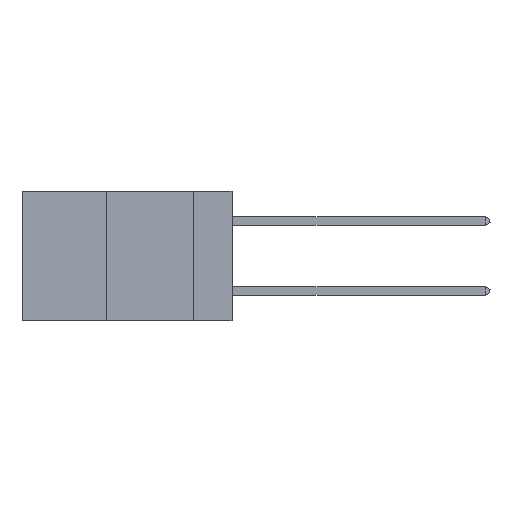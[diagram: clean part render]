
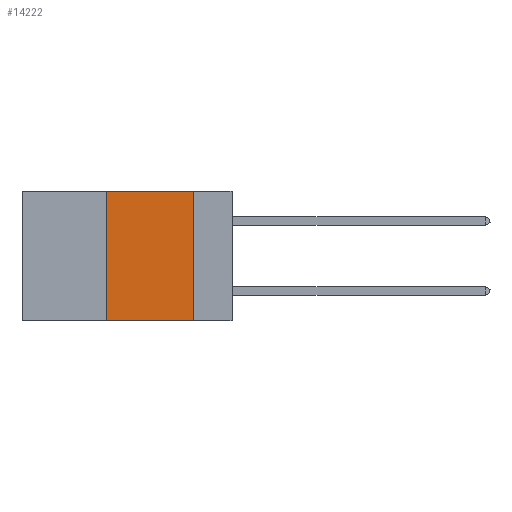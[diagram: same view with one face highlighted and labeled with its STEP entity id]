
A CAD part, left-side view. The second image highlights one B-rep face of the part: STEP entity #14222.
In plain terms, the highlighted planar face has unit normal (-1, 0, 0).
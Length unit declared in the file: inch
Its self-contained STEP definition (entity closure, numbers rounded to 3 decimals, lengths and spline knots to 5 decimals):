
#1043 = VECTOR ( 'NONE', #18296, 39.37008 ) ;
#1651 = CARTESIAN_POINT ( 'NONE',  ( 0., 0.11, 0. ) ) ;
#2403 = DIRECTION ( 'NONE',  ( 0., 0., 1. ) ) ;
#2477 = DIRECTION ( 'NONE',  ( 1., 0., 0. ) ) ;
#3644 = EDGE_CURVE ( 'NONE', #19221, #15955, #5813, .T. ) ;
#4206 = PLANE ( 'NONE',  #4920 ) ;
#4920 = AXIS2_PLACEMENT_3D ( 'NONE', #13035, #2477, #14788 ) ;
#5813 = LINE ( 'NONE', #13084, #1043 ) ;
#5834 = EDGE_CURVE ( 'NONE', #15955, #10063, #16811, .T. ) ;
#6502 = CARTESIAN_POINT ( 'NONE',  ( 0., 0.36, -0.37 ) ) ;
#8186 = DIRECTION ( 'NONE',  ( 0., -1., 0. ) ) ;
#8489 = VECTOR ( 'NONE', #2403, 39.37008 ) ;
#8500 = EDGE_CURVE ( 'NONE', #8532, #10063, #19958, .T. ) ;
#8532 = VERTEX_POINT ( 'NONE', #6502 ) ;
#8647 = VECTOR ( 'NONE', #9045, 39.37008 ) ;
#9045 = DIRECTION ( 'NONE',  ( 0., 0., -1. ) ) ;
#9354 = ORIENTED_EDGE ( 'NONE', *, *, #3644, .F. ) ;
#10063 = VERTEX_POINT ( 'NONE', #14155 ) ;
#11150 = ORIENTED_EDGE ( 'NONE', *, *, #5834, .F. ) ;
#11214 = CARTESIAN_POINT ( 'NONE',  ( 0., 0.36, 0. ) ) ;
#11793 = ORIENTED_EDGE ( 'NONE', *, *, #8500, .T. ) ;
#12041 = FACE_OUTER_BOUND ( 'NONE', #12995, .T. ) ;
#12995 = EDGE_LOOP ( 'NONE', ( #11150, #9354, #22563, #11793 ) ) ;
#13035 = CARTESIAN_POINT ( 'NONE',  ( 0., 0.6, 0. ) ) ;
#13084 = CARTESIAN_POINT ( 'NONE',  ( 0., 0.6, 0. ) ) ;
#14155 = CARTESIAN_POINT ( 'NONE',  ( 0., 0.11, -0.37 ) ) ;
#14199 = EDGE_CURVE ( 'NONE', #8532, #19221, #22297, .T. ) ;
#14222 = ADVANCED_FACE ( 'NONE', ( #12041 ), #4206, .F. ) ;
#14788 = DIRECTION ( 'NONE',  ( 0., 0., -1. ) ) ;
#15940 = VECTOR ( 'NONE', #8186, 39.37008 ) ;
#15955 = VERTEX_POINT ( 'NONE', #1651 ) ;
#16811 = LINE ( 'NONE', #21203, #8647 ) ;
#18296 = DIRECTION ( 'NONE',  ( 0., -1., 0. ) ) ;
#18586 = CARTESIAN_POINT ( 'NONE',  ( 0., 0.6, -0.37 ) ) ;
#19221 = VERTEX_POINT ( 'NONE', #20807 ) ;
#19958 = LINE ( 'NONE', #18586, #15940 ) ;
#20807 = CARTESIAN_POINT ( 'NONE',  ( 0., 0.36, 0. ) ) ;
#21203 = CARTESIAN_POINT ( 'NONE',  ( 0., 0.11, 0. ) ) ;
#22297 = LINE ( 'NONE', #11214, #8489 ) ;
#22563 = ORIENTED_EDGE ( 'NONE', *, *, #14199, .F. ) ;
